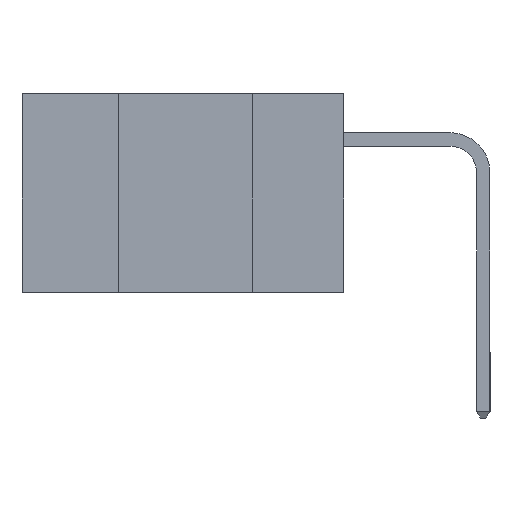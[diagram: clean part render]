
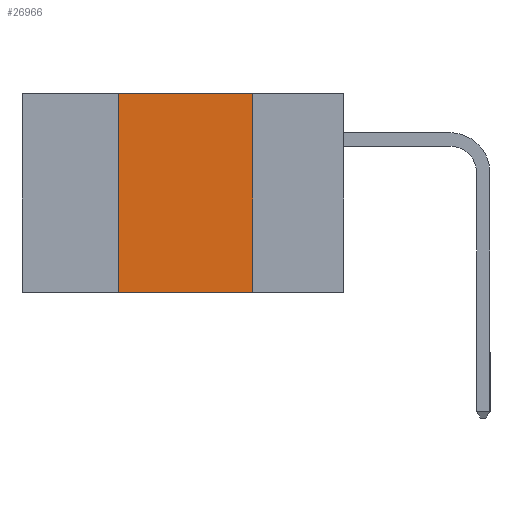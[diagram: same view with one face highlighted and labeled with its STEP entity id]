
A CAD part, left-side view. The second image highlights one B-rep face of the part: STEP entity #26966.
In plain terms, the highlighted planar face has unit normal (-1, 0, 0).
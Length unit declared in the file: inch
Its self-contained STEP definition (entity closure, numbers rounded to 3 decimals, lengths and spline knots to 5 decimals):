
#252 = DIRECTION ( 'NONE',  ( 0., -1., 0. ) ) ;
#639 = ORIENTED_EDGE ( 'NONE', *, *, #1750, .F. ) ;
#1750 = EDGE_CURVE ( 'NONE', #4931, #2834, #17286, .T. ) ;
#2200 = CARTESIAN_POINT ( 'NONE',  ( 0., 0.17, 0. ) ) ;
#2610 = VERTEX_POINT ( 'NONE', #23337 ) ;
#2834 = VERTEX_POINT ( 'NONE', #14270 ) ;
#3646 = LINE ( 'NONE', #11913, #20818 ) ;
#3677 = CARTESIAN_POINT ( 'NONE',  ( 0., 0.17, 0. ) ) ;
#4034 = VECTOR ( 'NONE', #252, 39.37008 ) ;
#4931 = VERTEX_POINT ( 'NONE', #2200 ) ;
#5296 = EDGE_CURVE ( 'NONE', #8050, #2610, #3646, .T. ) ;
#5350 = DIRECTION ( 'NONE',  ( 0., 0., -1. ) ) ;
#7660 = CARTESIAN_POINT ( 'NONE',  ( 0., 0.6, 0. ) ) ;
#7711 = VECTOR ( 'NONE', #8232, 39.37008 ) ;
#8050 = VERTEX_POINT ( 'NONE', #19301 ) ;
#8232 = DIRECTION ( 'NONE',  ( 0., 0., -1. ) ) ;
#8965 = AXIS2_PLACEMENT_3D ( 'NONE', #15189, #15387, #5350 ) ;
#8986 = CARTESIAN_POINT ( 'NONE',  ( 0., 0.6, -0.37 ) ) ;
#9682 = FACE_OUTER_BOUND ( 'NONE', #24921, .T. ) ;
#11913 = CARTESIAN_POINT ( 'NONE',  ( 0., 0.42, 0. ) ) ;
#12229 = DIRECTION ( 'NONE',  ( 0., 0., 1. ) ) ;
#12331 = ORIENTED_EDGE ( 'NONE', *, *, #21717, .F. ) ;
#14270 = CARTESIAN_POINT ( 'NONE',  ( 0., 0.17, -0.37 ) ) ;
#15189 = CARTESIAN_POINT ( 'NONE',  ( 0., 0.6, 0. ) ) ;
#15387 = DIRECTION ( 'NONE',  ( 1., 0., 0. ) ) ;
#17286 = LINE ( 'NONE', #3677, #7711 ) ;
#18543 = ORIENTED_EDGE ( 'NONE', *, *, #21016, .T. ) ;
#19301 = CARTESIAN_POINT ( 'NONE',  ( 0., 0.42, -0.37 ) ) ;
#20818 = VECTOR ( 'NONE', #12229, 39.37008 ) ;
#21016 = EDGE_CURVE ( 'NONE', #8050, #2834, #21281, .T. ) ;
#21281 = LINE ( 'NONE', #8986, #30291 ) ;
#21717 = EDGE_CURVE ( 'NONE', #2610, #4931, #29518, .T. ) ;
#23337 = CARTESIAN_POINT ( 'NONE',  ( 0., 0.42, 0. ) ) ;
#24762 = ORIENTED_EDGE ( 'NONE', *, *, #5296, .F. ) ;
#24921 = EDGE_LOOP ( 'NONE', ( #639, #12331, #24762, #18543 ) ) ;
#25590 = DIRECTION ( 'NONE',  ( 0., -1., 0. ) ) ;
#26966 = ADVANCED_FACE ( 'NONE', ( #9682 ), #27268, .F. ) ;
#27268 = PLANE ( 'NONE',  #8965 ) ;
#29518 = LINE ( 'NONE', #7660, #4034 ) ;
#30291 = VECTOR ( 'NONE', #25590, 39.37008 ) ;
